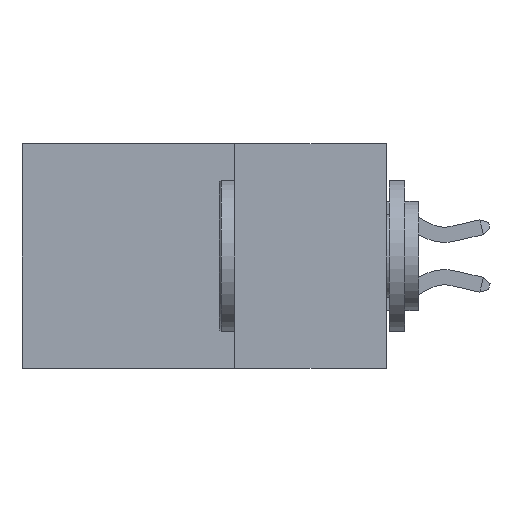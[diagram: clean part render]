
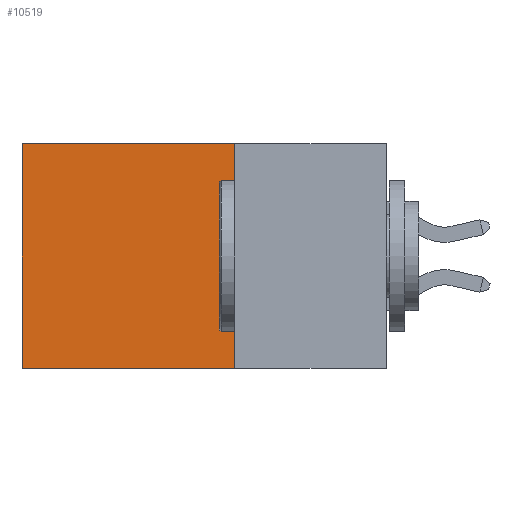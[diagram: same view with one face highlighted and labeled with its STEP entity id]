
A CAD part, left-side view. The second image highlights one B-rep face of the part: STEP entity #10519.
In plain terms, the highlighted planar face has unit normal (-1, 0, 0).
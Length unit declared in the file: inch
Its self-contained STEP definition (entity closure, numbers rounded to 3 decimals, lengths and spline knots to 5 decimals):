
#521 = CARTESIAN_POINT ( 'NONE',  ( 0.2615, 0.25, -0.37 ) ) ;
#1114 = VECTOR ( 'NONE', #9862, 39.37008 ) ;
#1398 = EDGE_CURVE ( 'NONE', #10642, #10275, #11782, .T. ) ;
#1714 = VECTOR ( 'NONE', #4030, 39.37008 ) ;
#2022 = CARTESIAN_POINT ( 'NONE',  ( 0.2615, 0.25, -0.37 ) ) ;
#3138 = VECTOR ( 'NONE', #10185, 39.37008 ) ;
#3179 = VERTEX_POINT ( 'NONE', #3901 ) ;
#3365 = CARTESIAN_POINT ( 'NONE',  ( 0.2615, 0.25, -0.37 ) ) ;
#3604 = ORIENTED_EDGE ( 'NONE', *, *, #7348, .F. ) ;
#3901 = CARTESIAN_POINT ( 'NONE',  ( 0.2615, 0.25, 0. ) ) ;
#4030 = DIRECTION ( 'NONE',  ( 0., 1., 0. ) ) ;
#4109 = FACE_OUTER_BOUND ( 'NONE', #10539, .T. ) ;
#4209 = PLANE ( 'NONE',  #9428 ) ;
#4901 = DIRECTION ( 'NONE',  ( 0., 1., 0. ) ) ;
#4968 = VECTOR ( 'NONE', #4901, 39.37008 ) ;
#5289 = DIRECTION ( 'NONE',  ( 1., 0., 0. ) ) ;
#7348 = EDGE_CURVE ( 'NONE', #3179, #8704, #8757, .T. ) ;
#7466 = LINE ( 'NONE', #8338, #1714 ) ;
#7650 = CARTESIAN_POINT ( 'NONE',  ( 0.2615, 0.6, 0. ) ) ;
#7693 = CARTESIAN_POINT ( 'NONE',  ( 0.2615, 0.25, -0.37 ) ) ;
#8194 = LINE ( 'NONE', #521, #4968 ) ;
#8338 = CARTESIAN_POINT ( 'NONE',  ( 0.2615, 0.25, 0. ) ) ;
#8704 = VERTEX_POINT ( 'NONE', #7693 ) ;
#8757 = LINE ( 'NONE', #3365, #1114 ) ;
#9036 = EDGE_CURVE ( 'NONE', #8704, #10275, #8194, .T. ) ;
#9428 = AXIS2_PLACEMENT_3D ( 'NONE', #2022, #5289, #12855 ) ;
#9849 = CARTESIAN_POINT ( 'NONE',  ( 0.2615, 0.6, -0.37 ) ) ;
#9862 = DIRECTION ( 'NONE',  ( 0., 0., -1. ) ) ;
#9982 = ORIENTED_EDGE ( 'NONE', *, *, #13386, .T. ) ;
#10185 = DIRECTION ( 'NONE',  ( 0., 0., -1. ) ) ;
#10275 = VERTEX_POINT ( 'NONE', #11185 ) ;
#10519 = ADVANCED_FACE ( 'NONE', ( #4109 ), #4209, .F. ) ;
#10539 = EDGE_LOOP ( 'NONE', ( #12343, #11255, #3604, #9982 ) ) ;
#10642 = VERTEX_POINT ( 'NONE', #7650 ) ;
#11185 = CARTESIAN_POINT ( 'NONE',  ( 0.2615, 0.6, -0.37 ) ) ;
#11255 = ORIENTED_EDGE ( 'NONE', *, *, #9036, .F. ) ;
#11782 = LINE ( 'NONE', #9849, #3138 ) ;
#12343 = ORIENTED_EDGE ( 'NONE', *, *, #1398, .T. ) ;
#12855 = DIRECTION ( 'NONE',  ( 0., 0., -1. ) ) ;
#13386 = EDGE_CURVE ( 'NONE', #3179, #10642, #7466, .T. ) ;
